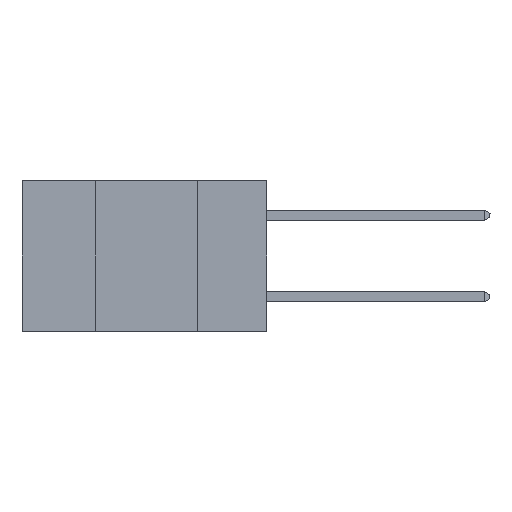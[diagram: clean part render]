
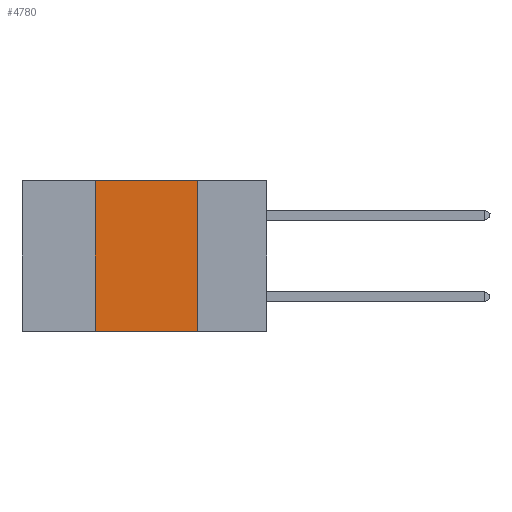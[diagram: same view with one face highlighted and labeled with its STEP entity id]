
A CAD part, left-side view. The second image highlights one B-rep face of the part: STEP entity #4780.
In plain terms, the highlighted planar face has unit normal (-1, 0, 0).
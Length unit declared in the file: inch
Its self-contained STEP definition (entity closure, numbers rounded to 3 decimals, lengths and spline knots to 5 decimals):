
#1217 = VERTEX_POINT ( 'NONE', #8334 ) ;
#1669 = VERTEX_POINT ( 'NONE', #12425 ) ;
#1891 = LINE ( 'NONE', #6685, #13995 ) ;
#1989 = LINE ( 'NONE', #4450, #10506 ) ;
#2040 = VERTEX_POINT ( 'NONE', #12664 ) ;
#2465 = DIRECTION ( 'NONE',  ( 1., 0., 0. ) ) ;
#3686 = AXIS2_PLACEMENT_3D ( 'NONE', #9468, #2465, #10545 ) ;
#4450 = CARTESIAN_POINT ( 'NONE',  ( 0., 0.42, 0. ) ) ;
#4780 = ADVANCED_FACE ( 'NONE', ( #7261 ), #14884, .F. ) ;
#5536 = DIRECTION ( 'NONE',  ( 0., 0., -1. ) ) ;
#5618 = DIRECTION ( 'NONE',  ( 0., 0., 1. ) ) ;
#5788 = EDGE_CURVE ( 'NONE', #2040, #1217, #6144, .T. ) ;
#6103 = LINE ( 'NONE', #9136, #14519 ) ;
#6144 = LINE ( 'NONE', #11093, #11653 ) ;
#6396 = CARTESIAN_POINT ( 'NONE',  ( 0., 0.42, 0. ) ) ;
#6685 = CARTESIAN_POINT ( 'NONE',  ( 0., 0.6, -0.37 ) ) ;
#7241 = EDGE_LOOP ( 'NONE', ( #8324, #8656, #11529, #14440 ) ) ;
#7261 = FACE_OUTER_BOUND ( 'NONE', #7241, .T. ) ;
#7821 = DIRECTION ( 'NONE',  ( 0., -1., 0. ) ) ;
#8090 = EDGE_CURVE ( 'NONE', #1669, #1217, #1891, .T. ) ;
#8324 = ORIENTED_EDGE ( 'NONE', *, *, #5788, .F. ) ;
#8334 = CARTESIAN_POINT ( 'NONE',  ( 0., 0.17, -0.37 ) ) ;
#8656 = ORIENTED_EDGE ( 'NONE', *, *, #11948, .F. ) ;
#8807 = EDGE_CURVE ( 'NONE', #1669, #12326, #1989, .T. ) ;
#9136 = CARTESIAN_POINT ( 'NONE',  ( 0., 0.6, 0. ) ) ;
#9468 = CARTESIAN_POINT ( 'NONE',  ( 0., 0.6, 0. ) ) ;
#10178 = DIRECTION ( 'NONE',  ( 0., -1., 0. ) ) ;
#10506 = VECTOR ( 'NONE', #5618, 39.37008 ) ;
#10545 = DIRECTION ( 'NONE',  ( 0., 0., -1. ) ) ;
#11093 = CARTESIAN_POINT ( 'NONE',  ( 0., 0.17, 0. ) ) ;
#11529 = ORIENTED_EDGE ( 'NONE', *, *, #8807, .F. ) ;
#11653 = VECTOR ( 'NONE', #5536, 39.37008 ) ;
#11948 = EDGE_CURVE ( 'NONE', #12326, #2040, #6103, .T. ) ;
#12326 = VERTEX_POINT ( 'NONE', #6396 ) ;
#12425 = CARTESIAN_POINT ( 'NONE',  ( 0., 0.42, -0.37 ) ) ;
#12664 = CARTESIAN_POINT ( 'NONE',  ( 0., 0.17, 0. ) ) ;
#13995 = VECTOR ( 'NONE', #7821, 39.37008 ) ;
#14440 = ORIENTED_EDGE ( 'NONE', *, *, #8090, .T. ) ;
#14519 = VECTOR ( 'NONE', #10178, 39.37008 ) ;
#14884 = PLANE ( 'NONE',  #3686 ) ;
